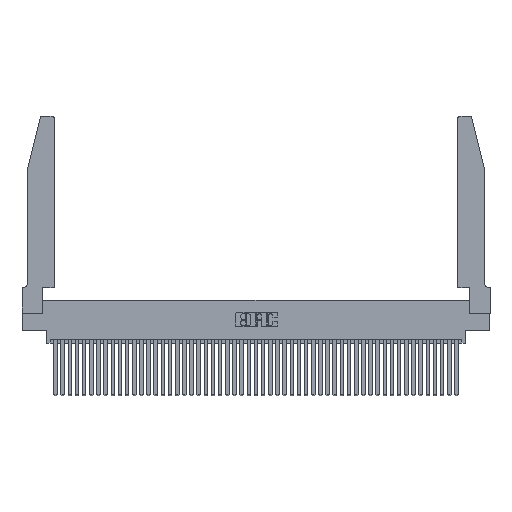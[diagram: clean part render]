
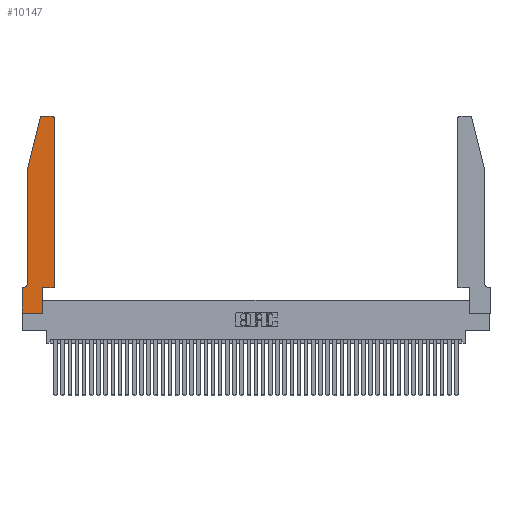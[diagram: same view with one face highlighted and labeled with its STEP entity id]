
A CAD part, top view. The second image highlights one B-rep face of the part: STEP entity #10147.
In plain terms, the highlighted planar face has unit normal (0, 0, 1).
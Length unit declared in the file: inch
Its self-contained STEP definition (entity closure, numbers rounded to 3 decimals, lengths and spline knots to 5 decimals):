
#503 = VECTOR ( 'NONE', #13901, 39.37008 ) ;
#1639 = LINE ( 'NONE', #43062, #31434 ) ;
#2506 = CARTESIAN_POINT ( 'NONE',  ( 0.284, 2.75, 0.37 ) ) ;
#2825 = LINE ( 'NONE', #24637, #503 ) ;
#3124 = CARTESIAN_POINT ( 'NONE',  ( 0.0055, 0.35, 0.37 ) ) ;
#3960 = DIRECTION ( 'NONE',  ( 0., 0., 1. ) ) ;
#4931 = ORIENTED_EDGE ( 'NONE', *, *, #36613, .T. ) ;
#5244 = ORIENTED_EDGE ( 'NONE', *, *, #35837, .T. ) ;
#5586 = EDGE_LOOP ( 'NONE', ( #5244, #42199, #17887, #34655, #19198, #23996, #46192, #17081, #23208, #4931, #30862, #26674 ) ) ;
#5667 = VECTOR ( 'NONE', #22582, 39.37008 ) ;
#5850 = LINE ( 'NONE', #27255, #27053 ) ;
#7033 = PLANE ( 'NONE',  #25827 ) ;
#7399 = VERTEX_POINT ( 'NONE', #29343 ) ;
#8801 = AXIS2_PLACEMENT_3D ( 'NONE', #37934, #41585, #37461 ) ;
#9909 = EDGE_CURVE ( 'NONE', #41628, #32923, #31092, .T. ) ;
#9953 = CARTESIAN_POINT ( 'NONE',  ( 0.2865, 0.35, 0.37 ) ) ;
#10147 = ADVANCED_FACE ( 'NONE', ( #43007 ), #7033, .T. ) ;
#12094 = EDGE_CURVE ( 'NONE', #20580, #44682, #42841, .T. ) ;
#12557 = CIRCLE ( 'NONE', #8801, 0.03 ) ;
#13428 = DIRECTION ( 'NONE',  ( 1., 0., 0. ) ) ;
#13687 = CARTESIAN_POINT ( 'NONE',  ( 0.0755, 0.42, 0.37 ) ) ;
#13901 = DIRECTION ( 'NONE',  ( -1., 0., 0. ) ) ;
#14121 = EDGE_CURVE ( 'NONE', #39864, #35154, #35557, .T. ) ;
#14323 = DIRECTION ( 'NONE',  ( 0., 0., 1. ) ) ;
#14559 = LINE ( 'NONE', #38844, #22034 ) ;
#15020 = EDGE_CURVE ( 'NONE', #35154, #7399, #12557, .T. ) ;
#15179 = CARTESIAN_POINT ( 'NONE',  ( 0.0755, 2., 0.37 ) ) ;
#16341 = DIRECTION ( 'NONE',  ( -1., 0., 0. ) ) ;
#17081 = ORIENTED_EDGE ( 'NONE', *, *, #17641, .T. ) ;
#17632 = EDGE_CURVE ( 'NONE', #43348, #18273, #24866, .T. ) ;
#17641 = EDGE_CURVE ( 'NONE', #18273, #20580, #14559, .T. ) ;
#17842 = DIRECTION ( 'NONE',  ( 1., 0., 0. ) ) ;
#17887 = ORIENTED_EDGE ( 'NONE', *, *, #35632, .T. ) ;
#18024 = DIRECTION ( 'NONE',  ( 1., 0., 0. ) ) ;
#18273 = VERTEX_POINT ( 'NONE', #42157 ) ;
#18395 = VERTEX_POINT ( 'NONE', #13687 ) ;
#19198 = ORIENTED_EDGE ( 'NONE', *, *, #26487, .T. ) ;
#20580 = VERTEX_POINT ( 'NONE', #43838 ) ;
#21949 = CARTESIAN_POINT ( 'NONE',  ( 0., 0.35, 0.37 ) ) ;
#22034 = VECTOR ( 'NONE', #13428, 39.37008 ) ;
#22582 = DIRECTION ( 'NONE',  ( 0., -1., 0. ) ) ;
#23208 = ORIENTED_EDGE ( 'NONE', *, *, #12094, .T. ) ;
#23744 = VECTOR ( 'NONE', #39002, 39.37008 ) ;
#23823 = EDGE_CURVE ( 'NONE', #30382, #43348, #5850, .T. ) ;
#23996 = ORIENTED_EDGE ( 'NONE', *, *, #23823, .T. ) ;
#24637 = CARTESIAN_POINT ( 'NONE',  ( 0.2605, 2.75, 0.37 ) ) ;
#24866 = LINE ( 'NONE', #35190, #23744 ) ;
#25666 = AXIS2_PLACEMENT_3D ( 'NONE', #28153, #46169, #42656 ) ;
#25782 = DIRECTION ( 'NONE',  ( 1., 0., 0. ) ) ;
#25827 = AXIS2_PLACEMENT_3D ( 'NONE', #21949, #3960, #25782 ) ;
#26487 = EDGE_CURVE ( 'NONE', #18395, #30382, #41023, .T. ) ;
#26674 = ORIENTED_EDGE ( 'NONE', *, *, #15020, .T. ) ;
#27053 = VECTOR ( 'NONE', #16341, 39.37008 ) ;
#27255 = CARTESIAN_POINT ( 'NONE',  ( 0.0755, 0.35, 0.37 ) ) ;
#27395 = DIRECTION ( 'NONE',  ( -0.239, -0.971, 0. ) ) ;
#27969 = EDGE_CURVE ( 'NONE', #43803, #18395, #44552, .T. ) ;
#28102 = VECTOR ( 'NONE', #27395, 39.37008 ) ;
#28153 = CARTESIAN_POINT ( 'NONE',  ( 0.0055, 0.42, 0.37 ) ) ;
#28382 = CARTESIAN_POINT ( 'NONE',  ( 0.4505, 2.72, 0.37 ) ) ;
#29343 = CARTESIAN_POINT ( 'NONE',  ( 0.4205, 2.75, 0.37 ) ) ;
#30382 = VERTEX_POINT ( 'NONE', #3124 ) ;
#30414 = LINE ( 'NONE', #38399, #28102 ) ;
#30750 = DIRECTION ( 'NONE',  ( 0., 1., 0. ) ) ;
#30862 = ORIENTED_EDGE ( 'NONE', *, *, #14121, .T. ) ;
#31092 = CIRCLE ( 'NONE', #37436, 0.03 ) ;
#31434 = VECTOR ( 'NONE', #17842, 39.37008 ) ;
#32923 = VERTEX_POINT ( 'NONE', #38913 ) ;
#33160 = VECTOR ( 'NONE', #30750, 39.37008 ) ;
#34655 = ORIENTED_EDGE ( 'NONE', *, *, #27969, .T. ) ;
#34698 = CARTESIAN_POINT ( 'NONE',  ( 0.0755, 2., 0.37 ) ) ;
#35154 = VERTEX_POINT ( 'NONE', #28382 ) ;
#35190 = CARTESIAN_POINT ( 'NONE',  ( 0., 0., 0.37 ) ) ;
#35557 = LINE ( 'NONE', #39426, #38990 ) ;
#35632 = EDGE_CURVE ( 'NONE', #32923, #43803, #30414, .T. ) ;
#35837 = EDGE_CURVE ( 'NONE', #7399, #41628, #2825, .T. ) ;
#36613 = EDGE_CURVE ( 'NONE', #44682, #39864, #1639, .T. ) ;
#37436 = AXIS2_PLACEMENT_3D ( 'NONE', #40053, #14323, #18024 ) ;
#37461 = DIRECTION ( 'NONE',  ( 1., 0., 0. ) ) ;
#37752 = CARTESIAN_POINT ( 'NONE',  ( 0.2865, 0.35, 0.37 ) ) ;
#37934 = CARTESIAN_POINT ( 'NONE',  ( 0.4205, 2.72, 0.37 ) ) ;
#38399 = CARTESIAN_POINT ( 'NONE',  ( 0.0755, 2., 0.37 ) ) ;
#38844 = CARTESIAN_POINT ( 'NONE',  ( 0., 0., 0.37 ) ) ;
#38913 = CARTESIAN_POINT ( 'NONE',  ( 0.25487, 2.72718, 0.37 ) ) ;
#38990 = VECTOR ( 'NONE', #43377, 39.37008 ) ;
#39002 = DIRECTION ( 'NONE',  ( 0., -1., 0. ) ) ;
#39426 = CARTESIAN_POINT ( 'NONE',  ( 0.4505, 0.35, 0.37 ) ) ;
#39864 = VERTEX_POINT ( 'NONE', #45984 ) ;
#40053 = CARTESIAN_POINT ( 'NONE',  ( 0.284, 2.72, 0.37 ) ) ;
#41023 = CIRCLE ( 'NONE', #25666, 0.07 ) ;
#41585 = DIRECTION ( 'NONE',  ( 0., 0., 1. ) ) ;
#41628 = VERTEX_POINT ( 'NONE', #2506 ) ;
#41906 = CARTESIAN_POINT ( 'NONE',  ( 0., 0.35, 0.37 ) ) ;
#42157 = CARTESIAN_POINT ( 'NONE',  ( 0., 0., 0.37 ) ) ;
#42199 = ORIENTED_EDGE ( 'NONE', *, *, #9909, .T. ) ;
#42656 = DIRECTION ( 'NONE',  ( -1., 0., 0. ) ) ;
#42841 = LINE ( 'NONE', #37752, #33160 ) ;
#43007 = FACE_OUTER_BOUND ( 'NONE', #5586, .T. ) ;
#43062 = CARTESIAN_POINT ( 'NONE',  ( 0.4505, 0.35, 0.37 ) ) ;
#43348 = VERTEX_POINT ( 'NONE', #41906 ) ;
#43377 = DIRECTION ( 'NONE',  ( 0., 1., 0. ) ) ;
#43803 = VERTEX_POINT ( 'NONE', #34698 ) ;
#43838 = CARTESIAN_POINT ( 'NONE',  ( 0.2865, 0., 0.37 ) ) ;
#44552 = LINE ( 'NONE', #15179, #5667 ) ;
#44682 = VERTEX_POINT ( 'NONE', #9953 ) ;
#45984 = CARTESIAN_POINT ( 'NONE',  ( 0.4505, 0.35, 0.37 ) ) ;
#46169 = DIRECTION ( 'NONE',  ( 0., 0., -1. ) ) ;
#46192 = ORIENTED_EDGE ( 'NONE', *, *, #17632, .T. ) ;
